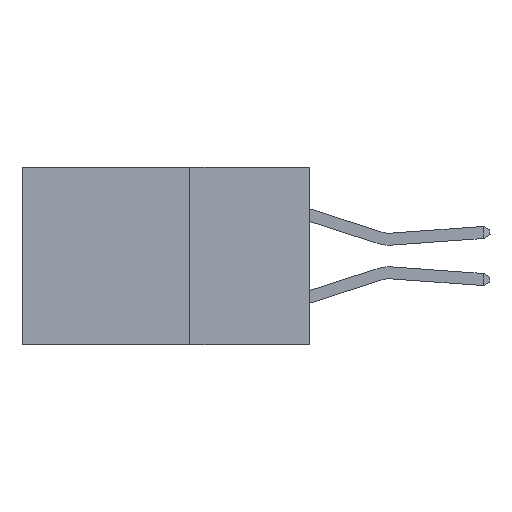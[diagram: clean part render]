
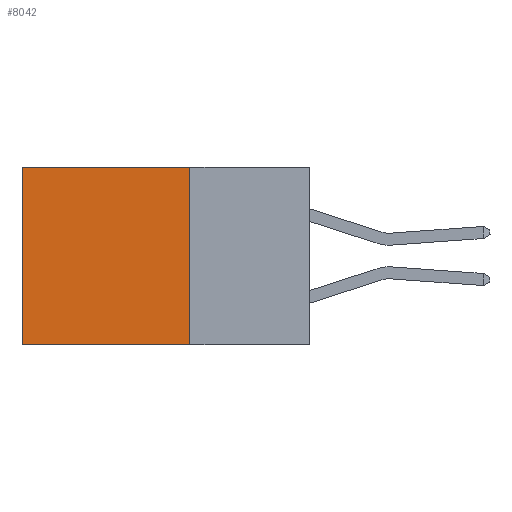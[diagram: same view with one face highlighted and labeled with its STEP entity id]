
A CAD part, left-side view. The second image highlights one B-rep face of the part: STEP entity #8042.
In plain terms, the highlighted planar face has unit normal (-1, 0, 0).
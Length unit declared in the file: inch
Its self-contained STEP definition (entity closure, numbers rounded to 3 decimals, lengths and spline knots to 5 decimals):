
#1003 = EDGE_CURVE ( 'NONE', #16752, #11339, #2691, .T. ) ;
#2130 = CARTESIAN_POINT ( 'NONE',  ( 0.298, 0.6, 0. ) ) ;
#2691 = LINE ( 'NONE', #9421, #9796 ) ;
#3056 = CARTESIAN_POINT ( 'NONE',  ( 0.298, 0.25, 0. ) ) ;
#3228 = VERTEX_POINT ( 'NONE', #10220 ) ;
#3553 = VECTOR ( 'NONE', #18204, 39.37008 ) ;
#3754 = EDGE_CURVE ( 'NONE', #3228, #8122, #11460, .T. ) ;
#4595 = DIRECTION ( 'NONE',  ( 0., 1., 0. ) ) ;
#6199 = DIRECTION ( 'NONE',  ( 0., 0., -1. ) ) ;
#7304 = EDGE_CURVE ( 'NONE', #8122, #11339, #11113, .T. ) ;
#7386 = VECTOR ( 'NONE', #6199, 39.37008 ) ;
#7734 = FACE_OUTER_BOUND ( 'NONE', #10952, .T. ) ;
#8042 = ADVANCED_FACE ( 'NONE', ( #7734 ), #16589, .F. ) ;
#8122 = VERTEX_POINT ( 'NONE', #12210 ) ;
#8193 = AXIS2_PLACEMENT_3D ( 'NONE', #13479, #19630, #10546 ) ;
#8512 = DIRECTION ( 'NONE',  ( 0., 0., -1. ) ) ;
#8969 = ORIENTED_EDGE ( 'NONE', *, *, #7304, .F. ) ;
#9392 = LINE ( 'NONE', #3056, #12973 ) ;
#9421 = CARTESIAN_POINT ( 'NONE',  ( 0.298, 0.6, 0. ) ) ;
#9768 = ORIENTED_EDGE ( 'NONE', *, *, #1003, .T. ) ;
#9796 = VECTOR ( 'NONE', #8512, 39.37008 ) ;
#10220 = CARTESIAN_POINT ( 'NONE',  ( 0.298, 0.25, 0. ) ) ;
#10546 = DIRECTION ( 'NONE',  ( 0., 0., -1. ) ) ;
#10765 = CARTESIAN_POINT ( 'NONE',  ( 0.298, 0.6, -0.37 ) ) ;
#10952 = EDGE_LOOP ( 'NONE', ( #9768, #8969, #16867, #16027 ) ) ;
#11113 = LINE ( 'NONE', #16681, #3553 ) ;
#11339 = VERTEX_POINT ( 'NONE', #10765 ) ;
#11460 = LINE ( 'NONE', #16750, #7386 ) ;
#12210 = CARTESIAN_POINT ( 'NONE',  ( 0.298, 0.25, -0.37 ) ) ;
#12973 = VECTOR ( 'NONE', #4595, 39.37008 ) ;
#13479 = CARTESIAN_POINT ( 'NONE',  ( 0.298, 0.25, 0. ) ) ;
#16027 = ORIENTED_EDGE ( 'NONE', *, *, #16502, .T. ) ;
#16502 = EDGE_CURVE ( 'NONE', #3228, #16752, #9392, .T. ) ;
#16589 = PLANE ( 'NONE',  #8193 ) ;
#16681 = CARTESIAN_POINT ( 'NONE',  ( 0.298, 0.25, -0.37 ) ) ;
#16750 = CARTESIAN_POINT ( 'NONE',  ( 0.298, 0.25, 0. ) ) ;
#16752 = VERTEX_POINT ( 'NONE', #2130 ) ;
#16867 = ORIENTED_EDGE ( 'NONE', *, *, #3754, .F. ) ;
#18204 = DIRECTION ( 'NONE',  ( 0., 1., 0. ) ) ;
#19630 = DIRECTION ( 'NONE',  ( 1., 0., 0. ) ) ;
